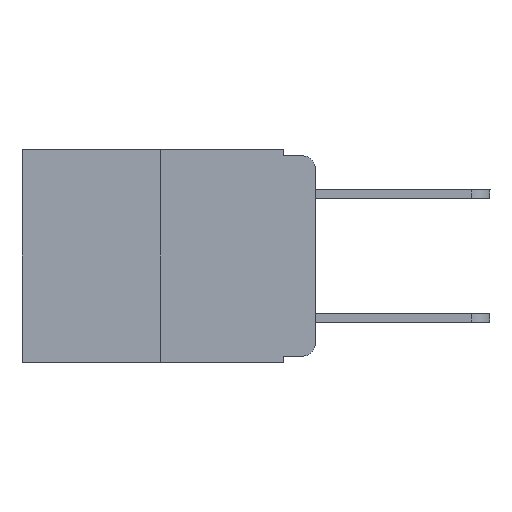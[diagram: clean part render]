
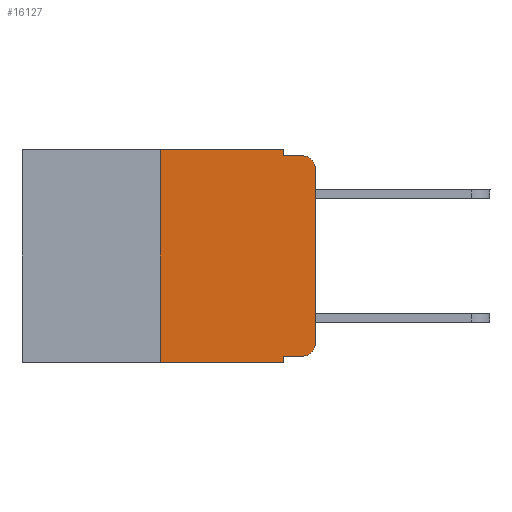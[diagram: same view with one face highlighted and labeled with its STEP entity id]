
A CAD part, left-side view. The second image highlights one B-rep face of the part: STEP entity #16127.
In plain terms, the highlighted planar face has unit normal (-1, 0, 0).
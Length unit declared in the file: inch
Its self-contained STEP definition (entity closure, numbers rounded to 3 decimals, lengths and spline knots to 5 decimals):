
#52 = EDGE_CURVE ( 'NONE', #14709, #6209, #6156, .T. ) ;
#112 = VERTEX_POINT ( 'NONE', #2520 ) ;
#215 = VECTOR ( 'NONE', #8978, 39.37008 ) ;
#297 = VERTEX_POINT ( 'NONE', #11953 ) ;
#918 = DIRECTION ( 'NONE',  ( 0., -1., 0. ) ) ;
#1315 = EDGE_CURVE ( 'NONE', #15239, #112, #5570, .T. ) ;
#1430 = ORIENTED_EDGE ( 'NONE', *, *, #4866, .F. ) ;
#1613 = VECTOR ( 'NONE', #9641, 39.37008 ) ;
#1771 = LINE ( 'NONE', #6806, #15279 ) ;
#1814 = DIRECTION ( 'NONE',  ( -1., 0., 0. ) ) ;
#1961 = DIRECTION ( 'NONE',  ( 0., -1., 0. ) ) ;
#2254 = EDGE_CURVE ( 'NONE', #14709, #15239, #1771, .T. ) ;
#2396 = CARTESIAN_POINT ( 'NONE',  ( 0., 0., 0. ) ) ;
#2457 = LINE ( 'NONE', #4787, #15933 ) ;
#2520 = CARTESIAN_POINT ( 'NONE',  ( 0., 0., -0.313 ) ) ;
#2590 = CARTESIAN_POINT ( 'NONE',  ( 0., 0.25, -0.343 ) ) ;
#2703 = EDGE_CURVE ( 'NONE', #4949, #6209, #2457, .T. ) ;
#3068 = CARTESIAN_POINT ( 'NONE',  ( 0., 0.051, 0. ) ) ;
#3069 = CARTESIAN_POINT ( 'NONE',  ( 0., 0.051, -0.333 ) ) ;
#3210 = CARTESIAN_POINT ( 'NONE',  ( 0., 0.02, -0.313 ) ) ;
#3395 = ORIENTED_EDGE ( 'NONE', *, *, #2254, .T. ) ;
#3610 = CARTESIAN_POINT ( 'NONE',  ( 0., 0.051, -0.01 ) ) ;
#3614 = DIRECTION ( 'NONE',  ( 0., -1., 0. ) ) ;
#3651 = ORIENTED_EDGE ( 'NONE', *, *, #7777, .F. ) ;
#3762 = VERTEX_POINT ( 'NONE', #3068 ) ;
#3776 = DIRECTION ( 'NONE',  ( 0., 0., -1. ) ) ;
#3936 = EDGE_LOOP ( 'NONE', ( #12248, #14281, #9926, #3651, #7655, #1430, #8253, #8296, #3395, #14930 ) ) ;
#4747 = DIRECTION ( 'NONE',  ( 0., 0., 1. ) ) ;
#4787 = CARTESIAN_POINT ( 'NONE',  ( 0., 0.473, -0.343 ) ) ;
#4809 = PLANE ( 'NONE',  #8193 ) ;
#4866 = EDGE_CURVE ( 'NONE', #4949, #297, #7368, .T. ) ;
#4949 = VERTEX_POINT ( 'NONE', #2590 ) ;
#5107 = CARTESIAN_POINT ( 'NONE',  ( 0., 0.02, -0.333 ) ) ;
#5374 = DIRECTION ( 'NONE',  ( 0., 0., -1. ) ) ;
#5570 = CIRCLE ( 'NONE', #8196, 0.02 ) ;
#6035 = DIRECTION ( 'NONE',  ( 0., 0., -1. ) ) ;
#6125 = FACE_OUTER_BOUND ( 'NONE', #3936, .T. ) ;
#6156 = LINE ( 'NONE', #16294, #15166 ) ;
#6209 = VERTEX_POINT ( 'NONE', #11703 ) ;
#6266 = CARTESIAN_POINT ( 'NONE',  ( 0., 0., -0.03 ) ) ;
#6597 = LINE ( 'NONE', #8806, #215 ) ;
#6806 = CARTESIAN_POINT ( 'NONE',  ( 0., 0.051, -0.333 ) ) ;
#6961 = VERTEX_POINT ( 'NONE', #6266 ) ;
#7107 = EDGE_CURVE ( 'NONE', #297, #3762, #6597, .T. ) ;
#7368 = LINE ( 'NONE', #16273, #16265 ) ;
#7655 = ORIENTED_EDGE ( 'NONE', *, *, #7107, .F. ) ;
#7777 = EDGE_CURVE ( 'NONE', #3762, #12595, #10957, .T. ) ;
#8193 = AXIS2_PLACEMENT_3D ( 'NONE', #14919, #13431, #6035 ) ;
#8196 = AXIS2_PLACEMENT_3D ( 'NONE', #3210, #1814, #5374 ) ;
#8253 = ORIENTED_EDGE ( 'NONE', *, *, #2703, .T. ) ;
#8296 = ORIENTED_EDGE ( 'NONE', *, *, #52, .F. ) ;
#8509 = LINE ( 'NONE', #2396, #1613 ) ;
#8806 = CARTESIAN_POINT ( 'NONE',  ( 0., 0.473, 0. ) ) ;
#8978 = DIRECTION ( 'NONE',  ( 0., -1., 0. ) ) ;
#9478 = VECTOR ( 'NONE', #1961, 39.37008 ) ;
#9641 = DIRECTION ( 'NONE',  ( 0., 0., 1. ) ) ;
#9679 = DIRECTION ( 'NONE',  ( 0., 0., -1. ) ) ;
#9848 = LINE ( 'NONE', #3610, #9478 ) ;
#9926 = ORIENTED_EDGE ( 'NONE', *, *, #13397, .F. ) ;
#10039 = VERTEX_POINT ( 'NONE', #12519 ) ;
#10724 = CARTESIAN_POINT ( 'NONE',  ( 0., 0.051, 0. ) ) ;
#10796 = CIRCLE ( 'NONE', #12882, 0.02 ) ;
#10957 = LINE ( 'NONE', #10724, #15254 ) ;
#11703 = CARTESIAN_POINT ( 'NONE',  ( 0., 0.051, -0.343 ) ) ;
#11953 = CARTESIAN_POINT ( 'NONE',  ( 0., 0.25, 0. ) ) ;
#12138 = CARTESIAN_POINT ( 'NONE',  ( 0., 0.02, -0.03 ) ) ;
#12248 = ORIENTED_EDGE ( 'NONE', *, *, #16218, .T. ) ;
#12519 = CARTESIAN_POINT ( 'NONE',  ( 0., 0.02, -0.01 ) ) ;
#12595 = VERTEX_POINT ( 'NONE', #14949 ) ;
#12882 = AXIS2_PLACEMENT_3D ( 'NONE', #12138, #13293, #9679 ) ;
#13293 = DIRECTION ( 'NONE',  ( -1., 0., 0. ) ) ;
#13397 = EDGE_CURVE ( 'NONE', #12595, #10039, #9848, .T. ) ;
#13431 = DIRECTION ( 'NONE',  ( 1., 0., 0. ) ) ;
#13705 = EDGE_CURVE ( 'NONE', #6961, #10039, #10796, .T. ) ;
#14281 = ORIENTED_EDGE ( 'NONE', *, *, #13705, .T. ) ;
#14709 = VERTEX_POINT ( 'NONE', #3069 ) ;
#14919 = CARTESIAN_POINT ( 'NONE',  ( 0., 0.473, 0. ) ) ;
#14930 = ORIENTED_EDGE ( 'NONE', *, *, #1315, .T. ) ;
#14949 = CARTESIAN_POINT ( 'NONE',  ( 0., 0.051, -0.01 ) ) ;
#15166 = VECTOR ( 'NONE', #3776, 39.37008 ) ;
#15239 = VERTEX_POINT ( 'NONE', #5107 ) ;
#15254 = VECTOR ( 'NONE', #16009, 39.37008 ) ;
#15279 = VECTOR ( 'NONE', #918, 39.37008 ) ;
#15933 = VECTOR ( 'NONE', #3614, 39.37008 ) ;
#16009 = DIRECTION ( 'NONE',  ( 0., 0., -1. ) ) ;
#16127 = ADVANCED_FACE ( 'NONE', ( #6125 ), #4809, .F. ) ;
#16218 = EDGE_CURVE ( 'NONE', #112, #6961, #8509, .T. ) ;
#16265 = VECTOR ( 'NONE', #4747, 39.37008 ) ;
#16273 = CARTESIAN_POINT ( 'NONE',  ( 0., 0.25, 0. ) ) ;
#16294 = CARTESIAN_POINT ( 'NONE',  ( 0., 0.051, 0. ) ) ;
